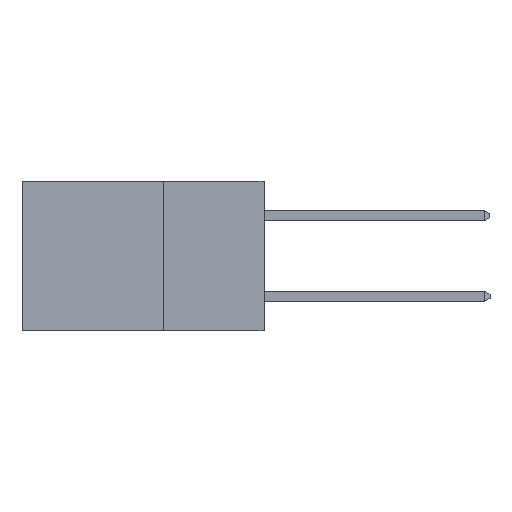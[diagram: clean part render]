
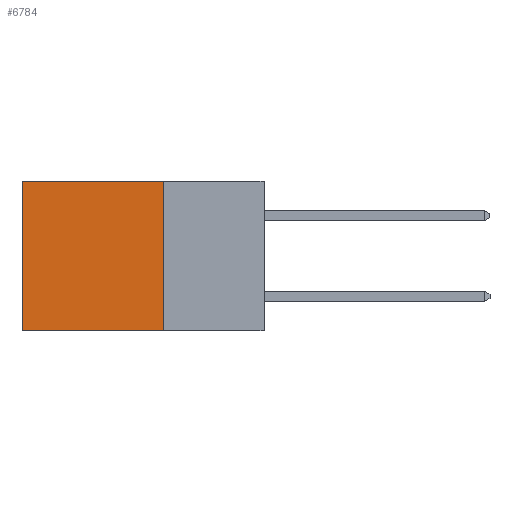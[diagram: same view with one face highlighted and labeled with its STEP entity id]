
A CAD part, left-side view. The second image highlights one B-rep face of the part: STEP entity #6784.
In plain terms, the highlighted planar face has unit normal (-1, 0, 0).
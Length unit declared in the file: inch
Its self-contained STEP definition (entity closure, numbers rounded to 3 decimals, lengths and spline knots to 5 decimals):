
#27 = DIRECTION ( 'NONE',  ( 0., 0., -1. ) ) ;
#120 = CARTESIAN_POINT ( 'NONE',  ( 0.2615, 0.6, -0.37 ) ) ;
#511 = EDGE_CURVE ( 'NONE', #8761, #1681, #2475, .T. ) ;
#697 = EDGE_CURVE ( 'NONE', #1828, #8761, #6991, .T. ) ;
#1001 = ORIENTED_EDGE ( 'NONE', *, *, #511, .T. ) ;
#1027 = AXIS2_PLACEMENT_3D ( 'NONE', #7085, #2660, #7781 ) ;
#1415 = CARTESIAN_POINT ( 'NONE',  ( 0.2615, 0.25, -0.37 ) ) ;
#1646 = CARTESIAN_POINT ( 'NONE',  ( 0.2615, 0.25, -0.37 ) ) ;
#1681 = VERTEX_POINT ( 'NONE', #6336 ) ;
#1699 = VERTEX_POINT ( 'NONE', #1415 ) ;
#1828 = VERTEX_POINT ( 'NONE', #4373 ) ;
#2089 = DIRECTION ( 'NONE',  ( 0., 1., 0. ) ) ;
#2389 = EDGE_LOOP ( 'NONE', ( #1001, #6820, #6776, #6243 ) ) ;
#2475 = LINE ( 'NONE', #120, #7866 ) ;
#2608 = LINE ( 'NONE', #4836, #4693 ) ;
#2660 = DIRECTION ( 'NONE',  ( 1., 0., 0. ) ) ;
#2963 = VECTOR ( 'NONE', #2089, 39.37008 ) ;
#4277 = CARTESIAN_POINT ( 'NONE',  ( 0.2615, 0.6, 0. ) ) ;
#4373 = CARTESIAN_POINT ( 'NONE',  ( 0.2615, 0.25, 0. ) ) ;
#4693 = VECTOR ( 'NONE', #4956, 39.37008 ) ;
#4836 = CARTESIAN_POINT ( 'NONE',  ( 0.2615, 0.25, -0.37 ) ) ;
#4956 = DIRECTION ( 'NONE',  ( 0., 0., -1. ) ) ;
#4973 = PLANE ( 'NONE',  #1027 ) ;
#5696 = EDGE_CURVE ( 'NONE', #1828, #1699, #2608, .T. ) ;
#5886 = EDGE_CURVE ( 'NONE', #1699, #1681, #7118, .T. ) ;
#6243 = ORIENTED_EDGE ( 'NONE', *, *, #697, .T. ) ;
#6336 = CARTESIAN_POINT ( 'NONE',  ( 0.2615, 0.6, -0.37 ) ) ;
#6549 = VECTOR ( 'NONE', #8734, 39.37008 ) ;
#6776 = ORIENTED_EDGE ( 'NONE', *, *, #5696, .F. ) ;
#6784 = ADVANCED_FACE ( 'NONE', ( #7101 ), #4973, .F. ) ;
#6820 = ORIENTED_EDGE ( 'NONE', *, *, #5886, .F. ) ;
#6991 = LINE ( 'NONE', #7989, #6549 ) ;
#7085 = CARTESIAN_POINT ( 'NONE',  ( 0.2615, 0.25, -0.37 ) ) ;
#7101 = FACE_OUTER_BOUND ( 'NONE', #2389, .T. ) ;
#7118 = LINE ( 'NONE', #1646, #2963 ) ;
#7781 = DIRECTION ( 'NONE',  ( 0., 0., -1. ) ) ;
#7866 = VECTOR ( 'NONE', #27, 39.37008 ) ;
#7989 = CARTESIAN_POINT ( 'NONE',  ( 0.2615, 0.25, 0. ) ) ;
#8734 = DIRECTION ( 'NONE',  ( 0., 1., 0. ) ) ;
#8761 = VERTEX_POINT ( 'NONE', #4277 ) ;
